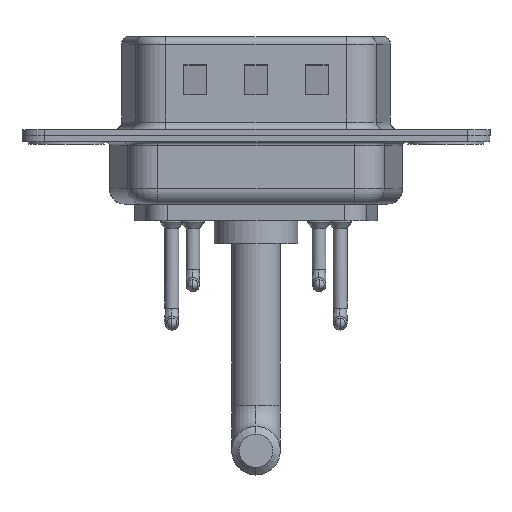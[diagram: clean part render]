
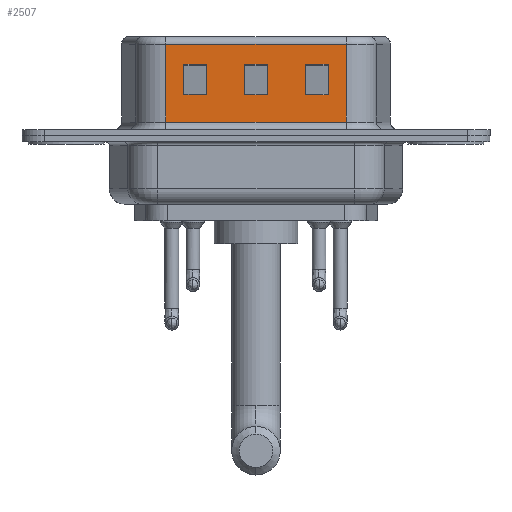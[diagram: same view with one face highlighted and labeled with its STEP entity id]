
A CAD part, front view. The second image highlights one B-rep face of the part: STEP entity #2507.
In plain terms, the highlighted planar face has unit normal (0, -1, 0).
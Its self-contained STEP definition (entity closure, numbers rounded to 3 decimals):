
#149 = EDGE_LOOP ( 'NONE', ( #12914, #9163, #1355, #14541 ) ) ;
#302 = CARTESIAN_POINT ( 'NONE',  ( 15.75, -4.55, 6.52 ) ) ;
#478 = CARTESIAN_POINT ( 'NONE',  ( 11.75, -4.55, 6.52 ) ) ;
#613 = LINE ( 'NONE', #1680, #8167 ) ;
#785 = EDGE_CURVE ( 'NONE', #12430, #15645, #1451, .T. ) ;
#930 = ORIENTED_EDGE ( 'NONE', *, *, #2790, .T. ) ;
#1099 = LINE ( 'NONE', #10941, #16281 ) ;
#1280 = VECTOR ( 'NONE', #12946, 1000. ) ;
#1355 = ORIENTED_EDGE ( 'NONE', *, *, #16651, .T. ) ;
#1451 = LINE ( 'NONE', #10869, #14985 ) ;
#1656 = FACE_OUTER_BOUND ( 'NONE', #149, .T. ) ;
#1680 = CARTESIAN_POINT ( 'NONE',  ( 18.451, -4.55, 4.705 ) ) ;
#1749 = ORIENTED_EDGE ( 'NONE', *, *, #11138, .T. ) ;
#1759 = FACE_BOUND ( 'NONE', #16210, .T. ) ;
#1866 = VECTOR ( 'NONE', #9119, 1000. ) ;
#1977 = VERTEX_POINT ( 'NONE', #15109 ) ;
#2088 = VERTEX_POINT ( 'NONE', #12422 ) ;
#2134 = CARTESIAN_POINT ( 'NONE',  ( 17.25, -4.55, 2.705 ) ) ;
#2315 = VERTEX_POINT ( 'NONE', #2452 ) ;
#2452 = CARTESIAN_POINT ( 'NONE',  ( 9.25, -4.55, 4.705 ) ) ;
#2496 = CARTESIAN_POINT ( 'NONE',  ( 13.25, -4.55, 6.52 ) ) ;
#2507 = ADVANCED_FACE ( 'NONE', ( #1759, #13818, #13928, #1656 ), #7060, .F. ) ;
#2735 = DIRECTION ( 'NONE',  ( 1., 0., 0. ) ) ;
#2765 = DIRECTION ( 'NONE',  ( -1., 0., 0. ) ) ;
#2779 = VECTOR ( 'NONE', #10213, 1000. ) ;
#2790 = EDGE_CURVE ( 'NONE', #1977, #10784, #613, .T. ) ;
#2837 = CARTESIAN_POINT ( 'NONE',  ( 18.451, -4.55, 0.9 ) ) ;
#2941 = DIRECTION ( 'NONE',  ( 0., 0., 1. ) ) ;
#3030 = DIRECTION ( 'NONE',  ( -1., 0., 0. ) ) ;
#3113 = ORIENTED_EDGE ( 'NONE', *, *, #11327, .T. ) ;
#3299 = CARTESIAN_POINT ( 'NONE',  ( 14.451, -4.55, 4.705 ) ) ;
#3389 = DIRECTION ( 'NONE',  ( 1., 0., 0. ) ) ;
#3465 = CARTESIAN_POINT ( 'NONE',  ( 6.549, -4.55, 6.52 ) ) ;
#3730 = EDGE_LOOP ( 'NONE', ( #3113, #1749, #4980, #6864 ) ) ;
#3839 = CARTESIAN_POINT ( 'NONE',  ( 18.451, -4.55, 0.9 ) ) ;
#4114 = ORIENTED_EDGE ( 'NONE', *, *, #14645, .T. ) ;
#4204 = VERTEX_POINT ( 'NONE', #2134 ) ;
#4253 = ORIENTED_EDGE ( 'NONE', *, *, #16062, .T. ) ;
#4320 = CARTESIAN_POINT ( 'NONE',  ( 7.75, -4.55, 2.705 ) ) ;
#4361 = LINE ( 'NONE', #8626, #12322 ) ;
#4454 = VERTEX_POINT ( 'NONE', #15802 ) ;
#4465 = DIRECTION ( 'NONE',  ( 0., 0., 1. ) ) ;
#4483 = CARTESIAN_POINT ( 'NONE',  ( 22.451, -4.55, 4.705 ) ) ;
#4840 = VECTOR ( 'NONE', #3389, 1000. ) ;
#4975 = DIRECTION ( 'NONE',  ( 0., 0., -1. ) ) ;
#4980 = ORIENTED_EDGE ( 'NONE', *, *, #14038, .T. ) ;
#5044 = VECTOR ( 'NONE', #12620, 1000. ) ;
#5124 = ORIENTED_EDGE ( 'NONE', *, *, #16695, .T. ) ;
#5136 = VERTEX_POINT ( 'NONE', #3839 ) ;
#5657 = DIRECTION ( 'NONE',  ( 1., 0., 0. ) ) ;
#5735 = DIRECTION ( 'NONE',  ( -1., 0., 0. ) ) ;
#5961 = VECTOR ( 'NONE', #7213, 1000. ) ;
#6310 = VERTEX_POINT ( 'NONE', #4320 ) ;
#6468 = VECTOR ( 'NONE', #10547, 1000. ) ;
#6790 = CARTESIAN_POINT ( 'NONE',  ( 6.549, -4.55, 6.02 ) ) ;
#6857 = EDGE_CURVE ( 'NONE', #4454, #5136, #17473, .T. ) ;
#6864 = ORIENTED_EDGE ( 'NONE', *, *, #14857, .T. ) ;
#6964 = DIRECTION ( 'NONE',  ( 0., 1., 0. ) ) ;
#6971 = ORIENTED_EDGE ( 'NONE', *, *, #10411, .T. ) ;
#7060 = PLANE ( 'NONE',  #10548 ) ;
#7213 = DIRECTION ( 'NONE',  ( 0., 0., 1. ) ) ;
#7309 = VERTEX_POINT ( 'NONE', #8221 ) ;
#7325 = CARTESIAN_POINT ( 'NONE',  ( 18.451, -4.55, 6.52 ) ) ;
#7518 = CARTESIAN_POINT ( 'NONE',  ( 9.25, -4.55, 6.52 ) ) ;
#7847 = LINE ( 'NONE', #13283, #6468 ) ;
#7917 = EDGE_CURVE ( 'NONE', #7309, #1977, #16642, .T. ) ;
#8167 = VECTOR ( 'NONE', #5657, 1000. ) ;
#8221 = CARTESIAN_POINT ( 'NONE',  ( 11.75, -4.55, 2.705 ) ) ;
#8360 = CARTESIAN_POINT ( 'NONE',  ( 18.451, -4.55, 6.02 ) ) ;
#8626 = CARTESIAN_POINT ( 'NONE',  ( 18.451, -4.55, 2.705 ) ) ;
#8760 = CARTESIAN_POINT ( 'NONE',  ( 9.25, -4.55, 2.705 ) ) ;
#9093 = VECTOR ( 'NONE', #16838, 1000. ) ;
#9119 = DIRECTION ( 'NONE',  ( 0., 0., -1. ) ) ;
#9163 = ORIENTED_EDGE ( 'NONE', *, *, #785, .T. ) ;
#9404 = EDGE_CURVE ( 'NONE', #6310, #2088, #15401, .T. ) ;
#9790 = LINE ( 'NONE', #302, #5961 ) ;
#10042 = LINE ( 'NONE', #3299, #4840 ) ;
#10213 = DIRECTION ( 'NONE',  ( 0., 0., -1. ) ) ;
#10250 = VECTOR ( 'NONE', #2941, 1000. ) ;
#10411 = EDGE_CURVE ( 'NONE', #10784, #10765, #15826, .T. ) ;
#10547 = DIRECTION ( 'NONE',  ( 0., 0., -1. ) ) ;
#10548 = AXIS2_PLACEMENT_3D ( 'NONE', #7325, #6964, #5735 ) ;
#10609 = DIRECTION ( 'NONE',  ( -1., 0., 0. ) ) ;
#10765 = VERTEX_POINT ( 'NONE', #14954 ) ;
#10784 = VERTEX_POINT ( 'NONE', #16463 ) ;
#10869 = CARTESIAN_POINT ( 'NONE',  ( 18.451, -4.55, 6.02 ) ) ;
#10941 = CARTESIAN_POINT ( 'NONE',  ( 14.451, -4.55, 2.705 ) ) ;
#11050 = CARTESIAN_POINT ( 'NONE',  ( 15.75, -4.55, 4.705 ) ) ;
#11138 = EDGE_CURVE ( 'NONE', #4204, #14660, #13854, .T. ) ;
#11327 = EDGE_CURVE ( 'NONE', #12087, #4204, #15721, .T. ) ;
#11486 = ORIENTED_EDGE ( 'NONE', *, *, #16043, .T. ) ;
#11587 = VERTEX_POINT ( 'NONE', #8760 ) ;
#11836 = CARTESIAN_POINT ( 'NONE',  ( 17.25, -4.55, 4.705 ) ) ;
#12071 = CARTESIAN_POINT ( 'NONE',  ( 15.75, -4.55, 2.705 ) ) ;
#12087 = VERTEX_POINT ( 'NONE', #11836 ) ;
#12322 = VECTOR ( 'NONE', #3030, 1000. ) ;
#12422 = CARTESIAN_POINT ( 'NONE',  ( 7.75, -4.55, 4.705 ) ) ;
#12430 = VERTEX_POINT ( 'NONE', #8360 ) ;
#12620 = DIRECTION ( 'NONE',  ( -1., 0., 0. ) ) ;
#12800 = CARTESIAN_POINT ( 'NONE',  ( 22.451, -4.55, 2.705 ) ) ;
#12914 = ORIENTED_EDGE ( 'NONE', *, *, #13250, .F. ) ;
#12946 = DIRECTION ( 'NONE',  ( 0., 0., -1. ) ) ;
#13250 = EDGE_CURVE ( 'NONE', #12430, #5136, #7847, .T. ) ;
#13283 = CARTESIAN_POINT ( 'NONE',  ( 18.451, -4.55, 6.52 ) ) ;
#13622 = ORIENTED_EDGE ( 'NONE', *, *, #9404, .T. ) ;
#13629 = VECTOR ( 'NONE', #4465, 1000. ) ;
#13818 = FACE_BOUND ( 'NONE', #3730, .T. ) ;
#13854 = LINE ( 'NONE', #12800, #5044 ) ;
#13928 = FACE_BOUND ( 'NONE', #15735, .T. ) ;
#13977 = CARTESIAN_POINT ( 'NONE',  ( 7.75, -4.55, 6.52 ) ) ;
#14038 = EDGE_CURVE ( 'NONE', #14660, #14084, #9790, .T. ) ;
#14084 = VERTEX_POINT ( 'NONE', #11050 ) ;
#14541 = ORIENTED_EDGE ( 'NONE', *, *, #6857, .T. ) ;
#14645 = EDGE_CURVE ( 'NONE', #2088, #2315, #10042, .T. ) ;
#14660 = VERTEX_POINT ( 'NONE', #12071 ) ;
#14857 = EDGE_CURVE ( 'NONE', #14084, #12087, #16658, .T. ) ;
#14954 = CARTESIAN_POINT ( 'NONE',  ( 13.25, -4.55, 2.705 ) ) ;
#14985 = VECTOR ( 'NONE', #2765, 1000. ) ;
#15109 = CARTESIAN_POINT ( 'NONE',  ( 11.75, -4.55, 4.705 ) ) ;
#15401 = LINE ( 'NONE', #13977, #10250 ) ;
#15627 = LINE ( 'NONE', #3465, #1866 ) ;
#15637 = CARTESIAN_POINT ( 'NONE',  ( 17.25, -4.55, 6.52 ) ) ;
#15645 = VERTEX_POINT ( 'NONE', #6790 ) ;
#15712 = LINE ( 'NONE', #7518, #1280 ) ;
#15721 = LINE ( 'NONE', #15637, #2779 ) ;
#15735 = EDGE_LOOP ( 'NONE', ( #930, #6971, #4253, #15954 ) ) ;
#15802 = CARTESIAN_POINT ( 'NONE',  ( 6.549, -4.55, 0.9 ) ) ;
#15826 = LINE ( 'NONE', #2496, #16793 ) ;
#15954 = ORIENTED_EDGE ( 'NONE', *, *, #7917, .T. ) ;
#16043 = EDGE_CURVE ( 'NONE', #11587, #6310, #1099, .T. ) ;
#16062 = EDGE_CURVE ( 'NONE', #10765, #7309, #4361, .T. ) ;
#16210 = EDGE_LOOP ( 'NONE', ( #5124, #11486, #13622, #4114 ) ) ;
#16281 = VECTOR ( 'NONE', #10609, 1000. ) ;
#16463 = CARTESIAN_POINT ( 'NONE',  ( 13.25, -4.55, 4.705 ) ) ;
#16642 = LINE ( 'NONE', #478, #13629 ) ;
#16651 = EDGE_CURVE ( 'NONE', #15645, #4454, #15627, .T. ) ;
#16658 = LINE ( 'NONE', #4483, #9093 ) ;
#16695 = EDGE_CURVE ( 'NONE', #2315, #11587, #15712, .T. ) ;
#16725 = VECTOR ( 'NONE', #2735, 1000. ) ;
#16793 = VECTOR ( 'NONE', #4975, 1000. ) ;
#16838 = DIRECTION ( 'NONE',  ( 1., 0., 0. ) ) ;
#17473 = LINE ( 'NONE', #2837, #16725 ) ;
